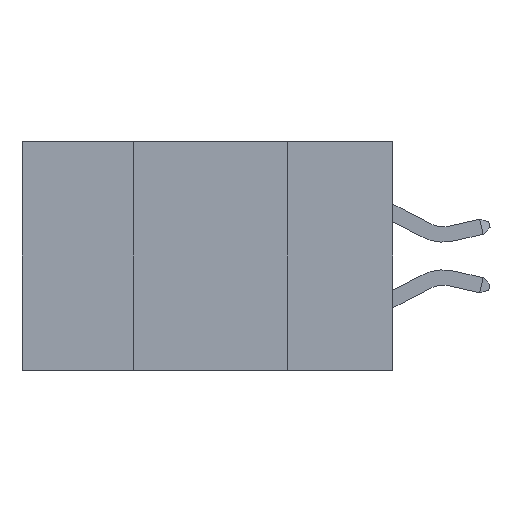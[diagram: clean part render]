
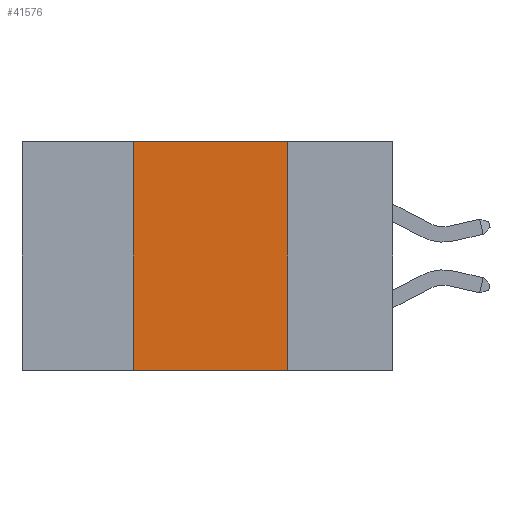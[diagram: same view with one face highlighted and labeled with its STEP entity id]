
A CAD part, left-side view. The second image highlights one B-rep face of the part: STEP entity #41576.
In plain terms, the highlighted planar face has unit normal (-1, 0, 0).
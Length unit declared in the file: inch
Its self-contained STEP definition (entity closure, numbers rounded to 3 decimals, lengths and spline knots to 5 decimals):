
#1496 = EDGE_LOOP ( 'NONE', ( #18695, #28973, #7714, #38926 ) ) ;
#3937 = VERTEX_POINT ( 'NONE', #36285 ) ;
#6606 = DIRECTION ( 'NONE',  ( 0., -1., 0. ) ) ;
#7012 = LINE ( 'NONE', #37430, #41736 ) ;
#7714 = ORIENTED_EDGE ( 'NONE', *, *, #10433, .F. ) ;
#7932 = PLANE ( 'NONE',  #31247 ) ;
#8374 = FACE_OUTER_BOUND ( 'NONE', #1496, .T. ) ;
#9675 = LINE ( 'NONE', #39871, #11428 ) ;
#10433 = EDGE_CURVE ( 'NONE', #3937, #22198, #7012, .T. ) ;
#11428 = VECTOR ( 'NONE', #20270, 39.37008 ) ;
#11448 = CARTESIAN_POINT ( 'NONE',  ( 0., 0.6, 0. ) ) ;
#12271 = CARTESIAN_POINT ( 'NONE',  ( 0., 0.17, -0.37 ) ) ;
#12348 = EDGE_CURVE ( 'NONE', #22198, #21053, #13383, .T. ) ;
#12772 = CARTESIAN_POINT ( 'NONE',  ( 0., 0.6, -0.37 ) ) ;
#12943 = DIRECTION ( 'NONE',  ( 0., -1., 0. ) ) ;
#13383 = LINE ( 'NONE', #23129, #28860 ) ;
#18695 = ORIENTED_EDGE ( 'NONE', *, *, #40570, .F. ) ;
#20270 = DIRECTION ( 'NONE',  ( 0., 0., -1. ) ) ;
#20476 = DIRECTION ( 'NONE',  ( 0., 0., 1. ) ) ;
#21053 = VERTEX_POINT ( 'NONE', #35028 ) ;
#22198 = VERTEX_POINT ( 'NONE', #34810 ) ;
#23129 = CARTESIAN_POINT ( 'NONE',  ( 0., 0.6, 0. ) ) ;
#24362 = VERTEX_POINT ( 'NONE', #12271 ) ;
#28860 = VECTOR ( 'NONE', #12943, 39.37008 ) ;
#28973 = ORIENTED_EDGE ( 'NONE', *, *, #12348, .F. ) ;
#31247 = AXIS2_PLACEMENT_3D ( 'NONE', #11448, #38575, #35059 ) ;
#31651 = EDGE_CURVE ( 'NONE', #3937, #24362, #36379, .T. ) ;
#34810 = CARTESIAN_POINT ( 'NONE',  ( 0., 0.42, 0. ) ) ;
#35028 = CARTESIAN_POINT ( 'NONE',  ( 0., 0.17, 0. ) ) ;
#35059 = DIRECTION ( 'NONE',  ( 0., 0., -1. ) ) ;
#35665 = VECTOR ( 'NONE', #6606, 39.37008 ) ;
#36285 = CARTESIAN_POINT ( 'NONE',  ( 0., 0.42, -0.37 ) ) ;
#36379 = LINE ( 'NONE', #12772, #35665 ) ;
#37430 = CARTESIAN_POINT ( 'NONE',  ( 0., 0.42, 0. ) ) ;
#38575 = DIRECTION ( 'NONE',  ( 1., 0., 0. ) ) ;
#38926 = ORIENTED_EDGE ( 'NONE', *, *, #31651, .T. ) ;
#39871 = CARTESIAN_POINT ( 'NONE',  ( 0., 0.17, 0. ) ) ;
#40570 = EDGE_CURVE ( 'NONE', #21053, #24362, #9675, .T. ) ;
#41576 = ADVANCED_FACE ( 'NONE', ( #8374 ), #7932, .F. ) ;
#41736 = VECTOR ( 'NONE', #20476, 39.37008 ) ;
